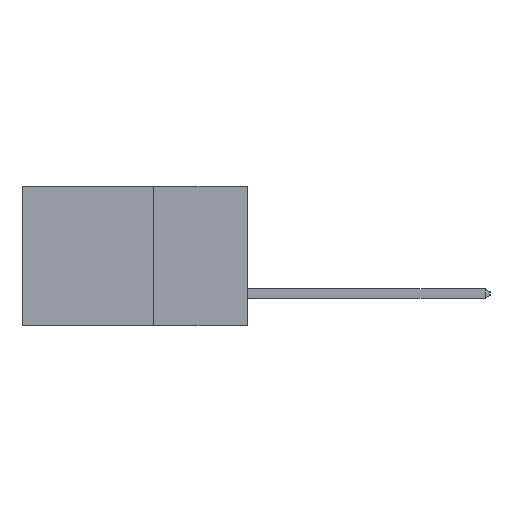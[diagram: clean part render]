
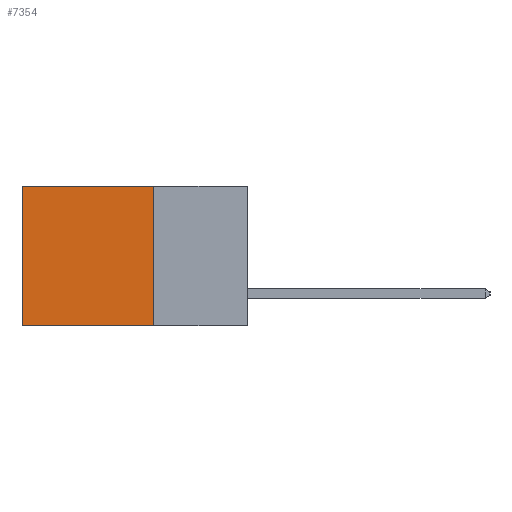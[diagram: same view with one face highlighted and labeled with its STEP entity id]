
A CAD part, left-side view. The second image highlights one B-rep face of the part: STEP entity #7354.
In plain terms, the highlighted planar face has unit normal (-1, 0, 0).
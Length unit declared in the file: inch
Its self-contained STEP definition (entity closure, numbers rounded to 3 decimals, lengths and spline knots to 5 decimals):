
#69 = ORIENTED_EDGE ( 'NONE', *, *, #650, .F. ) ;
#650 = EDGE_CURVE ( 'NONE', #22613, #4004, #2626, .T. ) ;
#845 = CARTESIAN_POINT ( 'NONE',  ( 0.298, 0.25, -0.37 ) ) ;
#2354 = VECTOR ( 'NONE', #9430, 39.37008 ) ;
#2544 = LINE ( 'NONE', #19577, #6886 ) ;
#2626 = LINE ( 'NONE', #845, #11827 ) ;
#4004 = VERTEX_POINT ( 'NONE', #21869 ) ;
#4492 = EDGE_CURVE ( 'NONE', #12605, #12468, #5008, .T. ) ;
#5008 = LINE ( 'NONE', #10842, #10467 ) ;
#5297 = CARTESIAN_POINT ( 'NONE',  ( 0.298, 0.25, 0. ) ) ;
#5748 = FACE_OUTER_BOUND ( 'NONE', #19122, .T. ) ;
#6886 = VECTOR ( 'NONE', #19391, 39.37008 ) ;
#7354 = ADVANCED_FACE ( 'NONE', ( #5748 ), #21837, .F. ) ;
#7865 = ORIENTED_EDGE ( 'NONE', *, *, #13305, .F. ) ;
#8124 = EDGE_CURVE ( 'NONE', #12468, #4004, #2544, .T. ) ;
#8950 = ORIENTED_EDGE ( 'NONE', *, *, #4492, .T. ) ;
#9430 = DIRECTION ( 'NONE',  ( 0., 0., -1. ) ) ;
#10467 = VECTOR ( 'NONE', #19730, 39.37008 ) ;
#10842 = CARTESIAN_POINT ( 'NONE',  ( 0.298, 0.25, 0. ) ) ;
#11827 = VECTOR ( 'NONE', #17642, 39.37008 ) ;
#12468 = VERTEX_POINT ( 'NONE', #21556 ) ;
#12605 = VERTEX_POINT ( 'NONE', #5297 ) ;
#13305 = EDGE_CURVE ( 'NONE', #12605, #22613, #17090, .T. ) ;
#15084 = ORIENTED_EDGE ( 'NONE', *, *, #8124, .T. ) ;
#17090 = LINE ( 'NONE', #20519, #2354 ) ;
#17642 = DIRECTION ( 'NONE',  ( 0., 1., 0. ) ) ;
#17993 = CARTESIAN_POINT ( 'NONE',  ( 0.298, 0.25, 0. ) ) ;
#19122 = EDGE_LOOP ( 'NONE', ( #15084, #69, #7865, #8950 ) ) ;
#19356 = CARTESIAN_POINT ( 'NONE',  ( 0.298, 0.25, -0.37 ) ) ;
#19391 = DIRECTION ( 'NONE',  ( 0., 0., -1. ) ) ;
#19577 = CARTESIAN_POINT ( 'NONE',  ( 0.298, 0.6, 0. ) ) ;
#19730 = DIRECTION ( 'NONE',  ( 0., 1., 0. ) ) ;
#20519 = CARTESIAN_POINT ( 'NONE',  ( 0.298, 0.25, 0. ) ) ;
#21419 = AXIS2_PLACEMENT_3D ( 'NONE', #17993, #21818, #22129 ) ;
#21556 = CARTESIAN_POINT ( 'NONE',  ( 0.298, 0.6, 0. ) ) ;
#21818 = DIRECTION ( 'NONE',  ( 1., 0., 0. ) ) ;
#21837 = PLANE ( 'NONE',  #21419 ) ;
#21869 = CARTESIAN_POINT ( 'NONE',  ( 0.298, 0.6, -0.37 ) ) ;
#22129 = DIRECTION ( 'NONE',  ( 0., 0., -1. ) ) ;
#22613 = VERTEX_POINT ( 'NONE', #19356 ) ;
